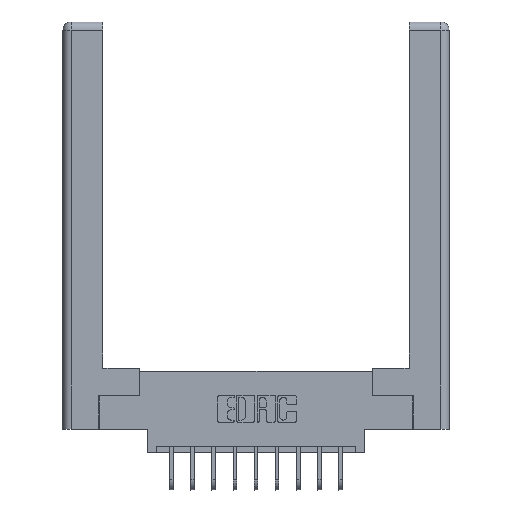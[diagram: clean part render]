
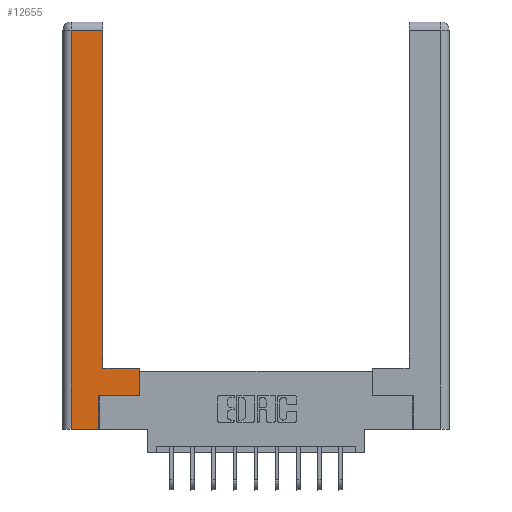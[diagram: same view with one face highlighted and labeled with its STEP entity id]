
A CAD part, top view. The second image highlights one B-rep face of the part: STEP entity #12655.
In plain terms, the highlighted planar face has unit normal (0, 0, 1).
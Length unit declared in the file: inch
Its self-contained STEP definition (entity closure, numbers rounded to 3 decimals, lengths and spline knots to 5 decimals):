
#44 = VECTOR ( 'NONE', #6686, 39.37008 ) ;
#126 = ORIENTED_EDGE ( 'NONE', *, *, #13609, .T. ) ;
#182 = CARTESIAN_POINT ( 'NONE',  ( 0.565, 0.245, 0. ) ) ;
#261 = ORIENTED_EDGE ( 'NONE', *, *, #6626, .T. ) ;
#413 = VERTEX_POINT ( 'NONE', #182 ) ;
#424 = VERTEX_POINT ( 'NONE', #7475 ) ;
#585 = CARTESIAN_POINT ( 'NONE',  ( 0.265, 0., 0. ) ) ;
#777 = EDGE_CURVE ( 'NONE', #13723, #13612, #5188, .T. ) ;
#1549 = CARTESIAN_POINT ( 'NONE',  ( 0.0615, 2.94, 0. ) ) ;
#1595 = DIRECTION ( 'NONE',  ( 0., -1., 0. ) ) ;
#2276 = CARTESIAN_POINT ( 'NONE',  ( 0.565, 0.245, 0. ) ) ;
#2515 = LINE ( 'NONE', #15142, #4957 ) ;
#2771 = VECTOR ( 'NONE', #6724, 39.37008 ) ;
#2852 = VERTEX_POINT ( 'NONE', #9668 ) ;
#3318 = ORIENTED_EDGE ( 'NONE', *, *, #777, .T. ) ;
#3547 = LINE ( 'NONE', #6828, #5057 ) ;
#3699 = DIRECTION ( 'NONE',  ( 0., 1., 0. ) ) ;
#3719 = VECTOR ( 'NONE', #7237, 39.37008 ) ;
#3842 = EDGE_CURVE ( 'NONE', #13612, #8800, #12858, .T. ) ;
#4037 = LINE ( 'NONE', #1549, #6518 ) ;
#4153 = VERTEX_POINT ( 'NONE', #8979 ) ;
#4320 = CARTESIAN_POINT ( 'NONE',  ( 0.0615, 0., 0. ) ) ;
#4787 = CARTESIAN_POINT ( 'NONE',  ( 0., 0., 0. ) ) ;
#4941 = EDGE_CURVE ( 'NONE', #2852, #413, #11564, .T. ) ;
#4957 = VECTOR ( 'NONE', #12752, 39.37008 ) ;
#5057 = VECTOR ( 'NONE', #6007, 39.37008 ) ;
#5083 = CARTESIAN_POINT ( 'NONE',  ( 0.265, 0., 0. ) ) ;
#5188 = LINE ( 'NONE', #7461, #7525 ) ;
#5560 = LINE ( 'NONE', #10820, #10973 ) ;
#6007 = DIRECTION ( 'NONE',  ( 0., 1., 0. ) ) ;
#6050 = FACE_OUTER_BOUND ( 'NONE', #13505, .T. ) ;
#6465 = ORIENTED_EDGE ( 'NONE', *, *, #13162, .T. ) ;
#6518 = VECTOR ( 'NONE', #8834, 39.37008 ) ;
#6626 = EDGE_CURVE ( 'NONE', #4153, #13723, #4037, .T. ) ;
#6686 = DIRECTION ( 'NONE',  ( 1., 0., 0. ) ) ;
#6724 = DIRECTION ( 'NONE',  ( -1., 0., 0. ) ) ;
#6828 = CARTESIAN_POINT ( 'NONE',  ( 0.295, 3., 0. ) ) ;
#7237 = DIRECTION ( 'NONE',  ( 1., 0., 0. ) ) ;
#7386 = ORIENTED_EDGE ( 'NONE', *, *, #3842, .T. ) ;
#7461 = CARTESIAN_POINT ( 'NONE',  ( 0.0615, 0., 0. ) ) ;
#7475 = CARTESIAN_POINT ( 'NONE',  ( 0.565, 0.45, 0. ) ) ;
#7514 = EDGE_CURVE ( 'NONE', #8800, #2852, #2515, .T. ) ;
#7525 = VECTOR ( 'NONE', #1595, 39.37008 ) ;
#7754 = ORIENTED_EDGE ( 'NONE', *, *, #7514, .T. ) ;
#7760 = AXIS2_PLACEMENT_3D ( 'NONE', #4787, #10872, #8008 ) ;
#8008 = DIRECTION ( 'NONE',  ( -1., 0., 0. ) ) ;
#8800 = VERTEX_POINT ( 'NONE', #5083 ) ;
#8834 = DIRECTION ( 'NONE',  ( -1., 0., 0. ) ) ;
#8979 = CARTESIAN_POINT ( 'NONE',  ( 0.295, 2.94, 0. ) ) ;
#9668 = CARTESIAN_POINT ( 'NONE',  ( 0.265, 0.245, 0. ) ) ;
#10820 = CARTESIAN_POINT ( 'NONE',  ( 0.565, 0.45, 0. ) ) ;
#10872 = DIRECTION ( 'NONE',  ( 0., 0., -1. ) ) ;
#10973 = VECTOR ( 'NONE', #3699, 39.37008 ) ;
#11096 = CARTESIAN_POINT ( 'NONE',  ( 0.295, 0.45, 0. ) ) ;
#11564 = LINE ( 'NONE', #2276, #3719 ) ;
#11619 = ORIENTED_EDGE ( 'NONE', *, *, #4941, .T. ) ;
#11888 = CARTESIAN_POINT ( 'NONE',  ( 0.0615, 2.94, 0. ) ) ;
#12362 = LINE ( 'NONE', #12869, #2771 ) ;
#12655 = ADVANCED_FACE ( 'NONE', ( #6050 ), #13302, .F. ) ;
#12752 = DIRECTION ( 'NONE',  ( 0., 1., 0. ) ) ;
#12858 = LINE ( 'NONE', #585, #44 ) ;
#12869 = CARTESIAN_POINT ( 'NONE',  ( 0.295, 0.45, 0. ) ) ;
#13162 = EDGE_CURVE ( 'NONE', #14025, #4153, #3547, .T. ) ;
#13302 = PLANE ( 'NONE',  #7760 ) ;
#13505 = EDGE_LOOP ( 'NONE', ( #6465, #261, #3318, #7386, #7754, #11619, #13937, #126 ) ) ;
#13609 = EDGE_CURVE ( 'NONE', #424, #14025, #12362, .T. ) ;
#13612 = VERTEX_POINT ( 'NONE', #4320 ) ;
#13723 = VERTEX_POINT ( 'NONE', #11888 ) ;
#13937 = ORIENTED_EDGE ( 'NONE', *, *, #14494, .T. ) ;
#14025 = VERTEX_POINT ( 'NONE', #11096 ) ;
#14494 = EDGE_CURVE ( 'NONE', #413, #424, #5560, .T. ) ;
#15142 = CARTESIAN_POINT ( 'NONE',  ( 0.265, 0.245, 0. ) ) ;
